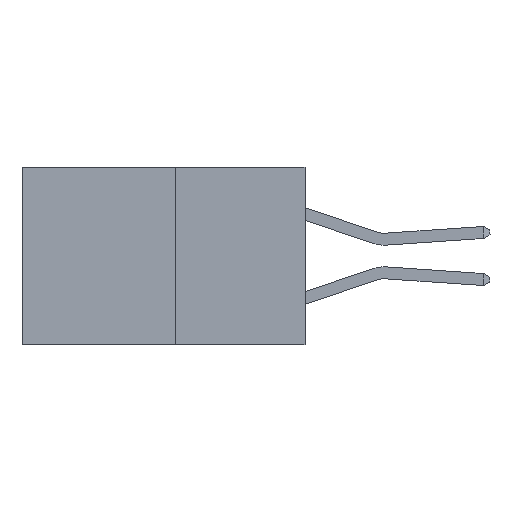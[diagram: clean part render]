
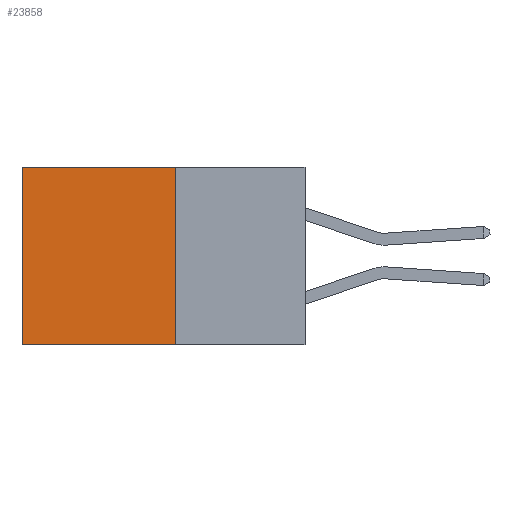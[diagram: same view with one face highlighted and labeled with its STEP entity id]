
A CAD part, left-side view. The second image highlights one B-rep face of the part: STEP entity #23858.
In plain terms, the highlighted planar face has unit normal (-1, 0, 0).
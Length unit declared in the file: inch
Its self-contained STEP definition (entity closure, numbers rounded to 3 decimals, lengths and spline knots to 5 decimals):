
#174 = VERTEX_POINT ( 'NONE', #16331 ) ;
#1240 = EDGE_LOOP ( 'NONE', ( #21646, #7757, #4990, #9748 ) ) ;
#1723 = VECTOR ( 'NONE', #18839, 39.37008 ) ;
#2408 = LINE ( 'NONE', #21014, #1723 ) ;
#3519 = CARTESIAN_POINT ( 'NONE',  ( 0.277, 0.27, -0.37 ) ) ;
#4894 = VECTOR ( 'NONE', #28357, 39.37008 ) ;
#4990 = ORIENTED_EDGE ( 'NONE', *, *, #10054, .F. ) ;
#5532 = PLANE ( 'NONE',  #22975 ) ;
#7737 = DIRECTION ( 'NONE',  ( 1., 0., 0. ) ) ;
#7757 = ORIENTED_EDGE ( 'NONE', *, *, #12309, .F. ) ;
#7884 = EDGE_CURVE ( 'NONE', #19378, #12266, #2408, .T. ) ;
#7920 = CARTESIAN_POINT ( 'NONE',  ( 0.277, 0.59, 0. ) ) ;
#8860 = VECTOR ( 'NONE', #12863, 39.37008 ) ;
#9541 = LINE ( 'NONE', #21578, #8860 ) ;
#9748 = ORIENTED_EDGE ( 'NONE', *, *, #24860, .T. ) ;
#10054 = EDGE_CURVE ( 'NONE', #174, #19748, #9541, .T. ) ;
#12086 = CARTESIAN_POINT ( 'NONE',  ( 0.277, 0.27, -0.37 ) ) ;
#12266 = VERTEX_POINT ( 'NONE', #23796 ) ;
#12309 = EDGE_CURVE ( 'NONE', #19748, #12266, #15923, .T. ) ;
#12863 = DIRECTION ( 'NONE',  ( 0., 0., -1. ) ) ;
#15923 = LINE ( 'NONE', #26139, #4894 ) ;
#16331 = CARTESIAN_POINT ( 'NONE',  ( 0.277, 0.27, 0. ) ) ;
#16505 = VECTOR ( 'NONE', #20173, 39.37008 ) ;
#17174 = LINE ( 'NONE', #17994, #16505 ) ;
#17994 = CARTESIAN_POINT ( 'NONE',  ( 0.277, 0.27, 0. ) ) ;
#18839 = DIRECTION ( 'NONE',  ( 0., 0., -1. ) ) ;
#19378 = VERTEX_POINT ( 'NONE', #7920 ) ;
#19748 = VERTEX_POINT ( 'NONE', #3519 ) ;
#20173 = DIRECTION ( 'NONE',  ( 0., 1., 0. ) ) ;
#21014 = CARTESIAN_POINT ( 'NONE',  ( 0.277, 0.59, -0.37 ) ) ;
#21347 = FACE_OUTER_BOUND ( 'NONE', #1240, .T. ) ;
#21578 = CARTESIAN_POINT ( 'NONE',  ( 0.277, 0.27, -0.37 ) ) ;
#21646 = ORIENTED_EDGE ( 'NONE', *, *, #7884, .T. ) ;
#22975 = AXIS2_PLACEMENT_3D ( 'NONE', #12086, #7737, #23113 ) ;
#23113 = DIRECTION ( 'NONE',  ( 0., 0., -1. ) ) ;
#23796 = CARTESIAN_POINT ( 'NONE',  ( 0.277, 0.59, -0.37 ) ) ;
#23858 = ADVANCED_FACE ( 'NONE', ( #21347 ), #5532, .F. ) ;
#24860 = EDGE_CURVE ( 'NONE', #174, #19378, #17174, .T. ) ;
#26139 = CARTESIAN_POINT ( 'NONE',  ( 0.277, 0.27, -0.37 ) ) ;
#28357 = DIRECTION ( 'NONE',  ( 0., 1., 0. ) ) ;
